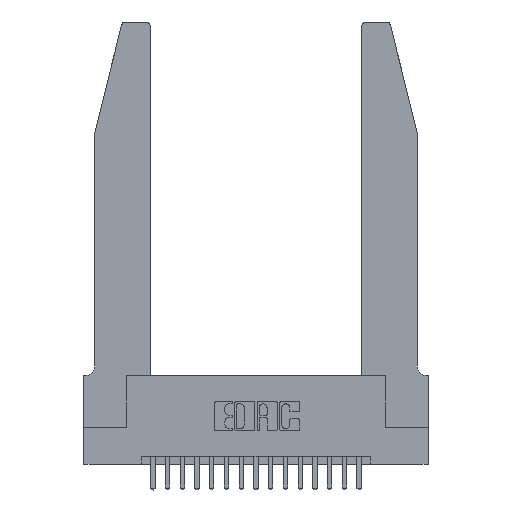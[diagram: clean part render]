
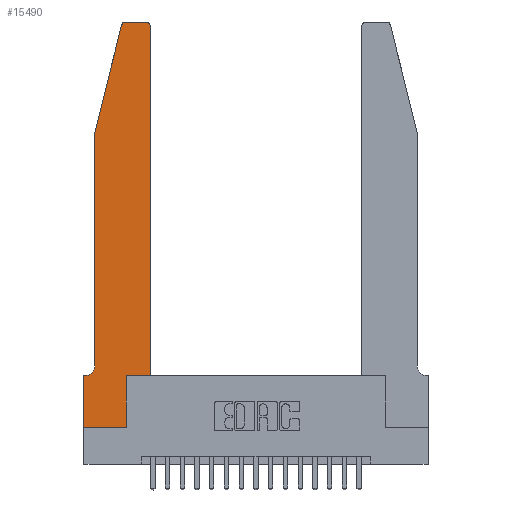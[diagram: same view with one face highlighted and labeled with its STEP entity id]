
A CAD part, top view. The second image highlights one B-rep face of the part: STEP entity #15490.
In plain terms, the highlighted planar face has unit normal (0, 0, 1).
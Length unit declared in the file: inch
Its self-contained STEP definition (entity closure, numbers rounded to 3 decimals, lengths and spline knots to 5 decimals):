
#380 = CARTESIAN_POINT ( 'NONE',  ( 0.2865, 0.35, 0.37 ) ) ;
#434 = LINE ( 'NONE', #17900, #3116 ) ;
#991 = CIRCLE ( 'NONE', #6083, 0.03 ) ;
#1047 = VERTEX_POINT ( 'NONE', #14130 ) ;
#1072 = DIRECTION ( 'NONE',  ( 1., 0., 0. ) ) ;
#1250 = LINE ( 'NONE', #11909, #12724 ) ;
#1357 = DIRECTION ( 'NONE',  ( -0.239, -0.971, 0. ) ) ;
#1458 = DIRECTION ( 'NONE',  ( 1., 0., 0. ) ) ;
#1523 = EDGE_CURVE ( 'NONE', #17339, #1047, #991, .T. ) ;
#1540 = LINE ( 'NONE', #7858, #12269 ) ;
#1769 = CARTESIAN_POINT ( 'NONE',  ( 0.2865, 0.35, 0.37 ) ) ;
#1827 = DIRECTION ( 'NONE',  ( -1., 0., 0. ) ) ;
#1900 = ORIENTED_EDGE ( 'NONE', *, *, #11975, .T. ) ;
#2106 = FACE_OUTER_BOUND ( 'NONE', #16744, .T. ) ;
#2758 = AXIS2_PLACEMENT_3D ( 'NONE', #13981, #17239, #15223 ) ;
#3116 = VECTOR ( 'NONE', #9642, 39.37008 ) ;
#3356 = CARTESIAN_POINT ( 'NONE',  ( 0.4505, 0.35, 0.37 ) ) ;
#3621 = CARTESIAN_POINT ( 'NONE',  ( 0.0755, 2., 0.37 ) ) ;
#4214 = VERTEX_POINT ( 'NONE', #12195 ) ;
#4260 = EDGE_CURVE ( 'NONE', #13720, #8113, #6486, .T. ) ;
#4375 = CARTESIAN_POINT ( 'NONE',  ( 0.2865, 0., 0.37 ) ) ;
#4436 = DIRECTION ( 'NONE',  ( 0., 0., 1. ) ) ;
#4466 = DIRECTION ( 'NONE',  ( 0., 0., 1. ) ) ;
#5140 = CARTESIAN_POINT ( 'NONE',  ( 0.0755, 0.35, 0.37 ) ) ;
#5697 = VECTOR ( 'NONE', #13258, 39.37008 ) ;
#6031 = ORIENTED_EDGE ( 'NONE', *, *, #1523, .T. ) ;
#6074 = EDGE_CURVE ( 'NONE', #8113, #7050, #8378, .T. ) ;
#6083 = AXIS2_PLACEMENT_3D ( 'NONE', #16755, #19620, #1072 ) ;
#6330 = DIRECTION ( 'NONE',  ( 0., 1., 0. ) ) ;
#6334 = CARTESIAN_POINT ( 'NONE',  ( 0.4505, 0.35, 0.37 ) ) ;
#6386 = VECTOR ( 'NONE', #6330, 39.37008 ) ;
#6412 = DIRECTION ( 'NONE',  ( 0., -1., 0. ) ) ;
#6486 = CIRCLE ( 'NONE', #18100, 0.03 ) ;
#6586 = VERTEX_POINT ( 'NONE', #1769 ) ;
#6857 = ORIENTED_EDGE ( 'NONE', *, *, #8571, .T. ) ;
#6970 = CARTESIAN_POINT ( 'NONE',  ( 0.0755, 0.42, 0.37 ) ) ;
#7050 = VERTEX_POINT ( 'NONE', #3621 ) ;
#7739 = CIRCLE ( 'NONE', #2758, 0.07 ) ;
#7858 = CARTESIAN_POINT ( 'NONE',  ( 0., 0., 0.37 ) ) ;
#8113 = VERTEX_POINT ( 'NONE', #13466 ) ;
#8364 = LINE ( 'NONE', #6334, #12033 ) ;
#8378 = LINE ( 'NONE', #16842, #17968 ) ;
#8568 = VERTEX_POINT ( 'NONE', #4375 ) ;
#8571 = EDGE_CURVE ( 'NONE', #17025, #9136, #7739, .T. ) ;
#8670 = EDGE_CURVE ( 'NONE', #1047, #13720, #434, .T. ) ;
#8846 = ORIENTED_EDGE ( 'NONE', *, *, #17512, .T. ) ;
#8886 = CARTESIAN_POINT ( 'NONE',  ( 0.0055, 0.35, 0.37 ) ) ;
#8939 = CARTESIAN_POINT ( 'NONE',  ( 0., 0., 0.37 ) ) ;
#9089 = PLANE ( 'NONE',  #20165 ) ;
#9095 = CARTESIAN_POINT ( 'NONE',  ( 0., 0.35, 0.37 ) ) ;
#9136 = VERTEX_POINT ( 'NONE', #8886 ) ;
#9642 = DIRECTION ( 'NONE',  ( -1., 0., 0. ) ) ;
#10129 = ORIENTED_EDGE ( 'NONE', *, *, #20134, .T. ) ;
#11011 = EDGE_CURVE ( 'NONE', #6586, #4214, #8364, .T. ) ;
#11084 = ORIENTED_EDGE ( 'NONE', *, *, #12799, .T. ) ;
#11608 = CARTESIAN_POINT ( 'NONE',  ( 0.284, 2.75, 0.37 ) ) ;
#11742 = ORIENTED_EDGE ( 'NONE', *, *, #4260, .T. ) ;
#11785 = VERTEX_POINT ( 'NONE', #9095 ) ;
#11909 = CARTESIAN_POINT ( 'NONE',  ( 0., 0., 0.37 ) ) ;
#11975 = EDGE_CURVE ( 'NONE', #11785, #19524, #1540, .T. ) ;
#12033 = VECTOR ( 'NONE', #15609, 39.37008 ) ;
#12195 = CARTESIAN_POINT ( 'NONE',  ( 0.4505, 0.35, 0.37 ) ) ;
#12269 = VECTOR ( 'NONE', #6412, 39.37008 ) ;
#12710 = EDGE_CURVE ( 'NONE', #19524, #8568, #1250, .T. ) ;
#12724 = VECTOR ( 'NONE', #14904, 39.37008 ) ;
#12799 = EDGE_CURVE ( 'NONE', #7050, #17025, #16435, .T. ) ;
#13258 = DIRECTION ( 'NONE',  ( 0., 1., 0. ) ) ;
#13466 = CARTESIAN_POINT ( 'NONE',  ( 0.25487, 2.72718, 0.37 ) ) ;
#13514 = ORIENTED_EDGE ( 'NONE', *, *, #6074, .T. ) ;
#13720 = VERTEX_POINT ( 'NONE', #11608 ) ;
#13805 = CARTESIAN_POINT ( 'NONE',  ( 0.284, 2.72, 0.37 ) ) ;
#13981 = CARTESIAN_POINT ( 'NONE',  ( 0.0055, 0.42, 0.37 ) ) ;
#14130 = CARTESIAN_POINT ( 'NONE',  ( 0.4205, 2.75, 0.37 ) ) ;
#14255 = LINE ( 'NONE', #3356, #6386 ) ;
#14349 = VECTOR ( 'NONE', #1827, 39.37008 ) ;
#14721 = ORIENTED_EDGE ( 'NONE', *, *, #8670, .T. ) ;
#14904 = DIRECTION ( 'NONE',  ( 1., 0., 0. ) ) ;
#15041 = EDGE_CURVE ( 'NONE', #9136, #11785, #16559, .T. ) ;
#15173 = CARTESIAN_POINT ( 'NONE',  ( 0.0755, 2., 0.37 ) ) ;
#15223 = DIRECTION ( 'NONE',  ( -1., 0., 0. ) ) ;
#15335 = CARTESIAN_POINT ( 'NONE',  ( 0.4505, 2.72, 0.37 ) ) ;
#15383 = DIRECTION ( 'NONE',  ( 1., 0., 0. ) ) ;
#15439 = VECTOR ( 'NONE', #19991, 39.37008 ) ;
#15490 = ADVANCED_FACE ( 'NONE', ( #2106 ), #9089, .T. ) ;
#15609 = DIRECTION ( 'NONE',  ( 1., 0., 0. ) ) ;
#16435 = LINE ( 'NONE', #15173, #15439 ) ;
#16559 = LINE ( 'NONE', #5140, #14349 ) ;
#16744 = EDGE_LOOP ( 'NONE', ( #14721, #11742, #13514, #11084, #6857, #19931, #1900, #19721, #10129, #17065, #8846, #6031 ) ) ;
#16755 = CARTESIAN_POINT ( 'NONE',  ( 0.4205, 2.72, 0.37 ) ) ;
#16842 = CARTESIAN_POINT ( 'NONE',  ( 0.0755, 2., 0.37 ) ) ;
#17025 = VERTEX_POINT ( 'NONE', #6970 ) ;
#17065 = ORIENTED_EDGE ( 'NONE', *, *, #11011, .T. ) ;
#17239 = DIRECTION ( 'NONE',  ( 0., 0., -1. ) ) ;
#17339 = VERTEX_POINT ( 'NONE', #15335 ) ;
#17512 = EDGE_CURVE ( 'NONE', #4214, #17339, #14255, .T. ) ;
#17900 = CARTESIAN_POINT ( 'NONE',  ( 0.2605, 2.75, 0.37 ) ) ;
#17968 = VECTOR ( 'NONE', #1357, 39.37008 ) ;
#18100 = AXIS2_PLACEMENT_3D ( 'NONE', #13805, #4436, #15383 ) ;
#18225 = LINE ( 'NONE', #380, #5697 ) ;
#19524 = VERTEX_POINT ( 'NONE', #8939 ) ;
#19620 = DIRECTION ( 'NONE',  ( 0., 0., 1. ) ) ;
#19721 = ORIENTED_EDGE ( 'NONE', *, *, #12710, .T. ) ;
#19931 = ORIENTED_EDGE ( 'NONE', *, *, #15041, .T. ) ;
#19991 = DIRECTION ( 'NONE',  ( 0., -1., 0. ) ) ;
#20134 = EDGE_CURVE ( 'NONE', #8568, #6586, #18225, .T. ) ;
#20165 = AXIS2_PLACEMENT_3D ( 'NONE', #20233, #4466, #1458 ) ;
#20233 = CARTESIAN_POINT ( 'NONE',  ( 0., 0.35, 0.37 ) ) ;
